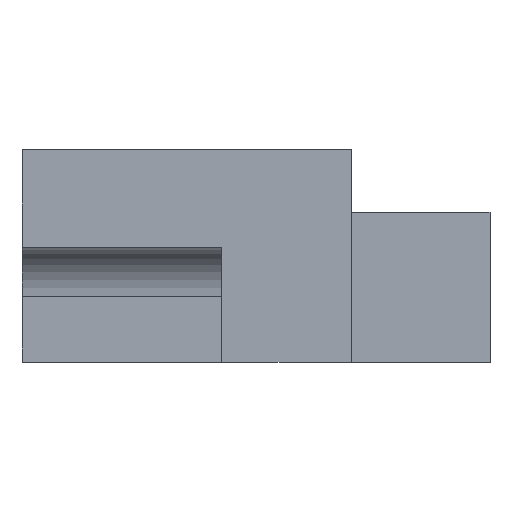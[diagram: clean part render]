
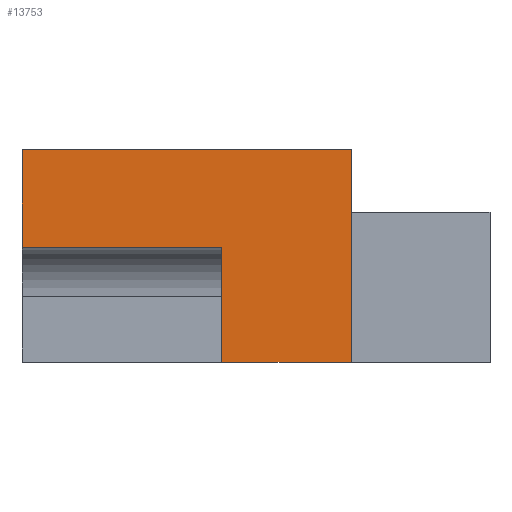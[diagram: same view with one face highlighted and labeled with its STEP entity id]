
A CAD part, left-side view. The second image highlights one B-rep face of the part: STEP entity #13753.
In plain terms, the highlighted planar face has unit normal (-1, 0, 0).
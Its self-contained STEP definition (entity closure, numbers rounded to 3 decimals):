
#509 = LINE ( 'NONE', #4783, #20396 ) ;
#1372 = CARTESIAN_POINT ( 'NONE',  ( 0., 8.255, -6.172 ) ) ;
#3142 = CARTESIAN_POINT ( 'NONE',  ( 0., 8.255, -6.172 ) ) ;
#3576 = CARTESIAN_POINT ( 'NONE',  ( 0., 20.955, 0. ) ) ;
#4156 = DIRECTION ( 'NONE',  ( 0., 0., 1. ) ) ;
#4744 = CARTESIAN_POINT ( 'NONE',  ( 0., 0., -13.487 ) ) ;
#4752 = VECTOR ( 'NONE', #4156, 1000. ) ;
#4783 = CARTESIAN_POINT ( 'NONE',  ( 0., 8.255, -13.487 ) ) ;
#4916 = ORIENTED_EDGE ( 'NONE', *, *, #27027, .F. ) ;
#5058 = EDGE_CURVE ( 'NONE', #26201, #16696, #31674, .T. ) ;
#5272 = EDGE_LOOP ( 'NONE', ( #6298, #12927, #29983, #18704, #4916, #25036 ) ) ;
#5279 = CARTESIAN_POINT ( 'NONE',  ( 0., 20.955, -6.172 ) ) ;
#5347 = LINE ( 'NONE', #5937, #29466 ) ;
#5937 = CARTESIAN_POINT ( 'NONE',  ( 0., -8.814, -13.487 ) ) ;
#5997 = VERTEX_POINT ( 'NONE', #3576 ) ;
#6298 = ORIENTED_EDGE ( 'NONE', *, *, #7987, .F. ) ;
#6569 = LINE ( 'NONE', #30712, #29170 ) ;
#7987 = EDGE_CURVE ( 'NONE', #16696, #20221, #5347, .T. ) ;
#8786 = DIRECTION ( 'NONE',  ( 0., 0., -1. ) ) ;
#11066 = DIRECTION ( 'NONE',  ( 0., 1., 0. ) ) ;
#11869 = CARTESIAN_POINT ( 'NONE',  ( 0., 0., 0. ) ) ;
#12179 = DIRECTION ( 'NONE',  ( 0., 0., 1. ) ) ;
#12415 = VERTEX_POINT ( 'NONE', #5279 ) ;
#12927 = ORIENTED_EDGE ( 'NONE', *, *, #5058, .F. ) ;
#13753 = ADVANCED_FACE ( 'NONE', ( #25991 ), #17804, .F. ) ;
#15660 = DIRECTION ( 'NONE',  ( 0., 1., 0. ) ) ;
#16639 = EDGE_CURVE ( 'NONE', #20221, #24486, #509, .T. ) ;
#16696 = VERTEX_POINT ( 'NONE', #4744 ) ;
#17079 = VECTOR ( 'NONE', #29080, 1000. ) ;
#17804 = PLANE ( 'NONE',  #27349 ) ;
#17881 = CARTESIAN_POINT ( 'NONE',  ( 0., 8.255, -13.487 ) ) ;
#18622 = EDGE_CURVE ( 'NONE', #5997, #26201, #6569, .T. ) ;
#18704 = ORIENTED_EDGE ( 'NONE', *, *, #28595, .F. ) ;
#19309 = LINE ( 'NONE', #28597, #4752 ) ;
#20221 = VERTEX_POINT ( 'NONE', #17881 ) ;
#20396 = VECTOR ( 'NONE', #12179, 1000. ) ;
#20897 = CARTESIAN_POINT ( 'NONE',  ( 0., 0., 0. ) ) ;
#24162 = CARTESIAN_POINT ( 'NONE',  ( 0., 0., 0. ) ) ;
#24486 = VERTEX_POINT ( 'NONE', #1372 ) ;
#25036 = ORIENTED_EDGE ( 'NONE', *, *, #16639, .F. ) ;
#25991 = FACE_OUTER_BOUND ( 'NONE', #5272, .T. ) ;
#26201 = VERTEX_POINT ( 'NONE', #11869 ) ;
#26951 = VECTOR ( 'NONE', #15660, 1000. ) ;
#27027 = EDGE_CURVE ( 'NONE', #24486, #12415, #27322, .T. ) ;
#27322 = LINE ( 'NONE', #3142, #26951 ) ;
#27349 = AXIS2_PLACEMENT_3D ( 'NONE', #20897, #30572, #8786 ) ;
#28595 = EDGE_CURVE ( 'NONE', #12415, #5997, #19309, .T. ) ;
#28597 = CARTESIAN_POINT ( 'NONE',  ( 0., 20.955, -13.487 ) ) ;
#29080 = DIRECTION ( 'NONE',  ( 0., 0., -1. ) ) ;
#29170 = VECTOR ( 'NONE', #29183, 1000. ) ;
#29183 = DIRECTION ( 'NONE',  ( 0., -1., 0. ) ) ;
#29466 = VECTOR ( 'NONE', #11066, 1000. ) ;
#29983 = ORIENTED_EDGE ( 'NONE', *, *, #18622, .F. ) ;
#30572 = DIRECTION ( 'NONE',  ( 1., 0., 0. ) ) ;
#30712 = CARTESIAN_POINT ( 'NONE',  ( 0., 11.506, 0. ) ) ;
#31674 = LINE ( 'NONE', #24162, #17079 ) ;
